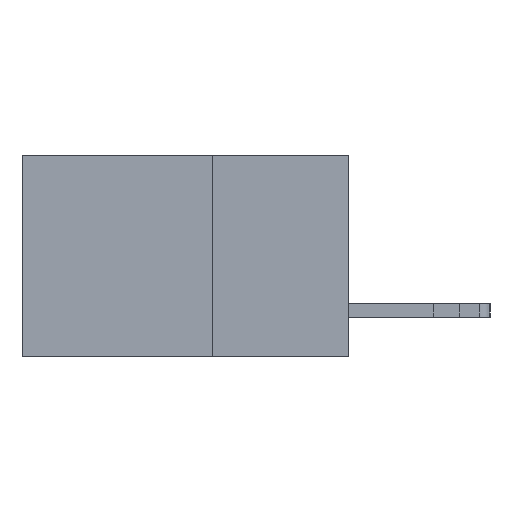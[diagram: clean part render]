
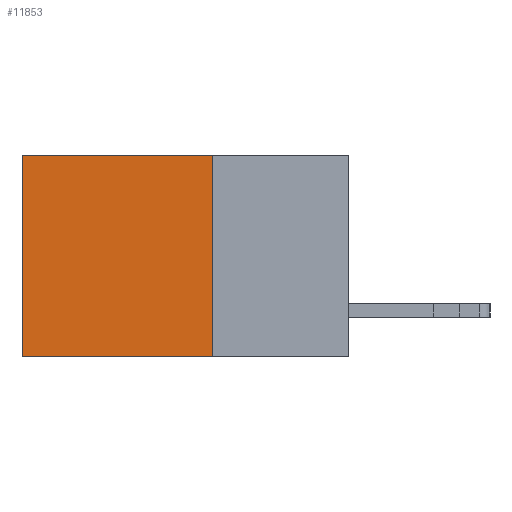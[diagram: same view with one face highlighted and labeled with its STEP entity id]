
A CAD part, left-side view. The second image highlights one B-rep face of the part: STEP entity #11853.
In plain terms, the highlighted planar face has unit normal (-1, 0, 0).
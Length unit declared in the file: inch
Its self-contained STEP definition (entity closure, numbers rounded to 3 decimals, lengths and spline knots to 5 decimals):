
#715 = LINE ( 'NONE', #5409, #3443 ) ;
#913 = CARTESIAN_POINT ( 'NONE',  ( 0.298, 0.6, 0. ) ) ;
#2173 = VECTOR ( 'NONE', #8824, 39.37008 ) ;
#2339 = LINE ( 'NONE', #6502, #8084 ) ;
#2631 = CARTESIAN_POINT ( 'NONE',  ( 0.298, 0.25, 0. ) ) ;
#2916 = EDGE_CURVE ( 'NONE', #10307, #9753, #4259, .T. ) ;
#2980 = CARTESIAN_POINT ( 'NONE',  ( 0.298, 0.6, -0.37 ) ) ;
#3211 = VERTEX_POINT ( 'NONE', #10701 ) ;
#3443 = VECTOR ( 'NONE', #9822, 39.37008 ) ;
#3452 = EDGE_CURVE ( 'NONE', #5628, #10307, #2339, .T. ) ;
#3913 = DIRECTION ( 'NONE',  ( 0., 0., -1. ) ) ;
#3956 = EDGE_CURVE ( 'NONE', #5628, #3211, #11225, .T. ) ;
#4226 = CARTESIAN_POINT ( 'NONE',  ( 0.298, 0.25, 0. ) ) ;
#4259 = LINE ( 'NONE', #913, #6167 ) ;
#5211 = AXIS2_PLACEMENT_3D ( 'NONE', #5595, #6704, #14461 ) ;
#5409 = CARTESIAN_POINT ( 'NONE',  ( 0.298, 0.25, -0.37 ) ) ;
#5595 = CARTESIAN_POINT ( 'NONE',  ( 0.298, 0.25, 0. ) ) ;
#5628 = VERTEX_POINT ( 'NONE', #2631 ) ;
#6167 = VECTOR ( 'NONE', #3913, 39.37008 ) ;
#6502 = CARTESIAN_POINT ( 'NONE',  ( 0.298, 0.25, 0. ) ) ;
#6704 = DIRECTION ( 'NONE',  ( 1., 0., 0. ) ) ;
#7821 = EDGE_LOOP ( 'NONE', ( #12874, #13267, #10608, #10368 ) ) ;
#8084 = VECTOR ( 'NONE', #8691, 39.37008 ) ;
#8532 = FACE_OUTER_BOUND ( 'NONE', #7821, .T. ) ;
#8691 = DIRECTION ( 'NONE',  ( 0., 1., 0. ) ) ;
#8824 = DIRECTION ( 'NONE',  ( 0., 0., -1. ) ) ;
#9753 = VERTEX_POINT ( 'NONE', #2980 ) ;
#9822 = DIRECTION ( 'NONE',  ( 0., 1., 0. ) ) ;
#10307 = VERTEX_POINT ( 'NONE', #12951 ) ;
#10368 = ORIENTED_EDGE ( 'NONE', *, *, #3452, .T. ) ;
#10608 = ORIENTED_EDGE ( 'NONE', *, *, #3956, .F. ) ;
#10701 = CARTESIAN_POINT ( 'NONE',  ( 0.298, 0.25, -0.37 ) ) ;
#11077 = EDGE_CURVE ( 'NONE', #3211, #9753, #715, .T. ) ;
#11225 = LINE ( 'NONE', #4226, #2173 ) ;
#11853 = ADVANCED_FACE ( 'NONE', ( #8532 ), #12273, .F. ) ;
#12273 = PLANE ( 'NONE',  #5211 ) ;
#12874 = ORIENTED_EDGE ( 'NONE', *, *, #2916, .T. ) ;
#12951 = CARTESIAN_POINT ( 'NONE',  ( 0.298, 0.6, 0. ) ) ;
#13267 = ORIENTED_EDGE ( 'NONE', *, *, #11077, .F. ) ;
#14461 = DIRECTION ( 'NONE',  ( 0., 0., -1. ) ) ;
